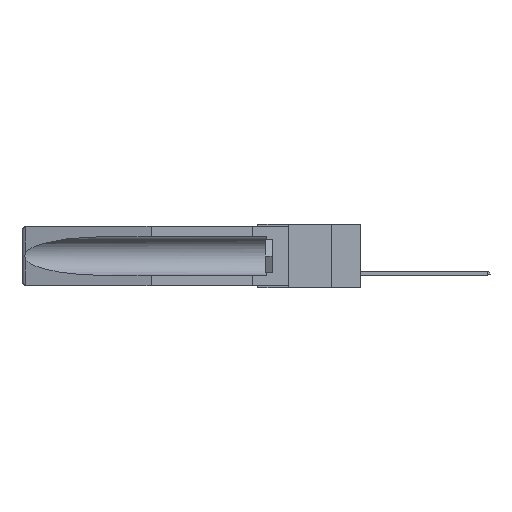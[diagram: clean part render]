
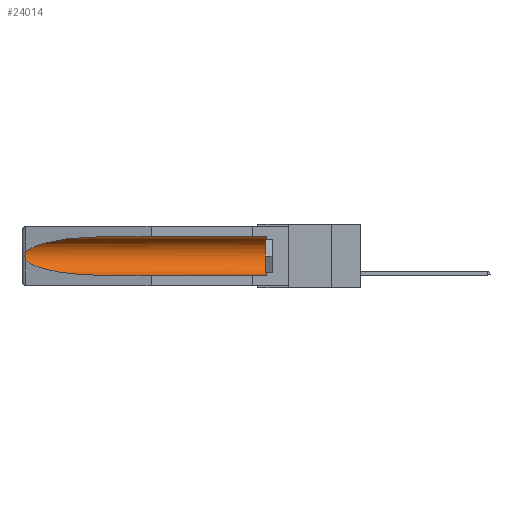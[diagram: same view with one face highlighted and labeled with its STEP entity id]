
A CAD part, left-side view. The second image highlights one B-rep face of the part: STEP entity #24014.
In plain terms, the highlighted cylindrical face has radius 2.857 mm (diameter 5.715 mm), a partial arc.
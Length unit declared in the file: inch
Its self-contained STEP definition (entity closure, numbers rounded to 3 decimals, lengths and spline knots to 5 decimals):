
#229 = DIRECTION ( 'NONE',  ( 0., 0., 1. ) ) ;
#352 = VERTEX_POINT ( 'NONE', #24342 ) ;
#1315 = CARTESIAN_POINT ( 'NONE',  ( 0.2675, 1.53308, -0.16763 ) ) ;
#1955 = CIRCLE ( 'NONE', #11311, 0.1125 ) ;
#2696 = EDGE_CURVE ( 'NONE', #8016, #14561, #1955, .T. ) ;
#2811 = VERTEX_POINT ( 'NONE', #21645 ) ;
#2891 = VECTOR ( 'NONE', #12562, 39.37008 ) ;
#3475 = EDGE_CURVE ( 'NONE', #14561, #7237, #21516, .T. ) ;
#4282 =( BOUNDED_CURVE ( )  B_SPLINE_CURVE ( 3, ( #11711, #13568, #7741, #21082 ),
 .UNSPECIFIED., .F., .F. ) 
 B_SPLINE_CURVE_WITH_KNOTS ( ( 4, 4 ),
 ( 0.1948, 1.5708 ),
 .UNSPECIFIED. ) 
 CURVE ( )  GEOMETRIC_REPRESENTATION_ITEM ( )  RATIONAL_B_SPLINE_CURVE ( ( 1., 0.848, 0.848, 1. ) ) 
 REPRESENTATION_ITEM ( '' )  );
#4822 = DIRECTION ( 'NONE',  ( 0., 1., 0. ) ) ;
#5224 = CARTESIAN_POINT ( 'NONE',  ( 0.26654, 1.53092, -0.15636 ) ) ;
#6961 = CARTESIAN_POINT ( 'NONE',  ( 0.26597, 1.52961, -0.15275 ) ) ;
#7237 = VERTEX_POINT ( 'NONE', #12558 ) ;
#7520 = CARTESIAN_POINT ( 'NONE',  ( 0.26537, 1.52718, -0.19328 ) ) ;
#7569 = CYLINDRICAL_SURFACE ( 'NONE', #14970, 0.1125 ) ;
#7741 = CARTESIAN_POINT ( 'NONE',  ( 0.21114, 1.30732, -0.284 ) ) ;
#7932 = CARTESIAN_POINT ( 'NONE',  ( 0.26537, 1.52718, -0.14972 ) ) ;
#8014 = ORIENTED_EDGE ( 'NONE', *, *, #13183, .F. ) ;
#8016 = VERTEX_POINT ( 'NONE', #9396 ) ;
#8720 = EDGE_LOOP ( 'NONE', ( #12244, #10895, #17031, #8014, #15367, #21052 ) ) ;
#8742 = CARTESIAN_POINT ( 'NONE',  ( 0.155, -0.30754, -0.1715 ) ) ;
#8748 = EDGE_CURVE ( 'NONE', #22158, #2811, #4282, .T. ) ;
#9396 = CARTESIAN_POINT ( 'NONE',  ( 0.155, 0.126, -0.284 ) ) ;
#10349 = LINE ( 'NONE', #12397, #2891 ) ;
#10740 = EDGE_CURVE ( 'NONE', #7237, #352, #23008, .T. ) ;
#10895 = ORIENTED_EDGE ( 'NONE', *, *, #13591, .T. ) ;
#11311 = AXIS2_PLACEMENT_3D ( 'NONE', #13645, #19499, #229 ) ;
#11711 = CARTESIAN_POINT ( 'NONE',  ( 0.26537, 1.52718, -0.19328 ) ) ;
#12244 = ORIENTED_EDGE ( 'NONE', *, *, #10740, .T. ) ;
#12385 = CARTESIAN_POINT ( 'NONE',  ( 0.155, 0.126, -0.059 ) ) ;
#12397 = CARTESIAN_POINT ( 'NONE',  ( 0.155, -0.30754, -0.284 ) ) ;
#12523 = CARTESIAN_POINT ( 'NONE',  ( 0.2673, 1.53269, -0.17917 ) ) ;
#12558 = CARTESIAN_POINT ( 'NONE',  ( 0.155, 1.07973, -0.059 ) ) ;
#12562 = DIRECTION ( 'NONE',  ( 0., 1., 0. ) ) ;
#12608 = CARTESIAN_POINT ( 'NONE',  ( 0.2675, 1.53308, -0.17534 ) ) ;
#13183 = EDGE_CURVE ( 'NONE', #8016, #2811, #10349, .T. ) ;
#13271 = CARTESIAN_POINT ( 'NONE',  ( 0.26597, 1.5296, -0.19026 ) ) ;
#13568 = CARTESIAN_POINT ( 'NONE',  ( 0.25451, 1.48313, -0.24835 ) ) ;
#13591 = EDGE_CURVE ( 'NONE', #352, #22158, #24511, .T. ) ;
#13645 = CARTESIAN_POINT ( 'NONE',  ( 0.155, 0.126, -0.1715 ) ) ;
#13914 = CARTESIAN_POINT ( 'NONE',  ( 0.25451, 1.48313, -0.09465 ) ) ;
#14290 = CARTESIAN_POINT ( 'NONE',  ( 0.26537, 1.52718, -0.19328 ) ) ;
#14561 = VERTEX_POINT ( 'NONE', #12385 ) ;
#14970 = AXIS2_PLACEMENT_3D ( 'NONE', #8742, #4822, #18186 ) ;
#15367 = ORIENTED_EDGE ( 'NONE', *, *, #2696, .T. ) ;
#15509 = CARTESIAN_POINT ( 'NONE',  ( 0.21114, 1.30732, -0.059 ) ) ;
#16172 = VECTOR ( 'NONE', #17488, 39.37008 ) ;
#17031 = ORIENTED_EDGE ( 'NONE', *, *, #8748, .T. ) ;
#17488 = DIRECTION ( 'NONE',  ( 0., 1., 0. ) ) ;
#18186 = DIRECTION ( 'NONE',  ( 0., 0., 1. ) ) ;
#18556 = FACE_OUTER_BOUND ( 'NONE', #8720, .T. ) ;
#18564 = CARTESIAN_POINT ( 'NONE',  ( 0.26537, 1.52718, -0.14972 ) ) ;
#19499 = DIRECTION ( 'NONE',  ( 0., -1., 0. ) ) ;
#19530 = CARTESIAN_POINT ( 'NONE',  ( 0.155, 1.07973, -0.059 ) ) ;
#20078 = CARTESIAN_POINT ( 'NONE',  ( 0.2673, 1.5327, -0.16383 ) ) ;
#20157 = CARTESIAN_POINT ( 'NONE',  ( 0.26655, 1.53094, -0.18657 ) ) ;
#21052 = ORIENTED_EDGE ( 'NONE', *, *, #3475, .T. ) ;
#21082 = CARTESIAN_POINT ( 'NONE',  ( 0.155, 1.07973, -0.284 ) ) ;
#21516 = LINE ( 'NONE', #23190, #16172 ) ;
#21645 = CARTESIAN_POINT ( 'NONE',  ( 0.155, 1.07973, -0.284 ) ) ;
#22158 = VERTEX_POINT ( 'NONE', #14290 ) ;
#23008 =( BOUNDED_CURVE ( )  B_SPLINE_CURVE ( 3, ( #19530, #15509, #13914, #7932 ),
 .UNSPECIFIED., .F., .F. ) 
 B_SPLINE_CURVE_WITH_KNOTS ( ( 4, 4 ),
 ( 4.71239, 6.08839 ),
 .UNSPECIFIED. ) 
 CURVE ( )  GEOMETRIC_REPRESENTATION_ITEM ( )  RATIONAL_B_SPLINE_CURVE ( ( 1., 0.848, 0.848, 1. ) ) 
 REPRESENTATION_ITEM ( '' )  );
#23190 = CARTESIAN_POINT ( 'NONE',  ( 0.155, -0.30754, -0.059 ) ) ;
#24014 = ADVANCED_FACE ( 'NONE', ( #18556 ), #7569, .F. ) ;
#24342 = CARTESIAN_POINT ( 'NONE',  ( 0.26537, 1.52718, -0.14972 ) ) ;
#24511 = B_SPLINE_CURVE_WITH_KNOTS ( 'NONE', 3,
 ( #18564, #6961, #5224, #20078, #1315, #12608, #12523, #20157, #13271, #7520 ),
 .UNSPECIFIED., .F., .F.,
 ( 4, 2, 2, 2, 4 ),
 ( 0., 0.00029, 0.00058, 0.00087, 0.00117 ),
 .UNSPECIFIED. ) ;
